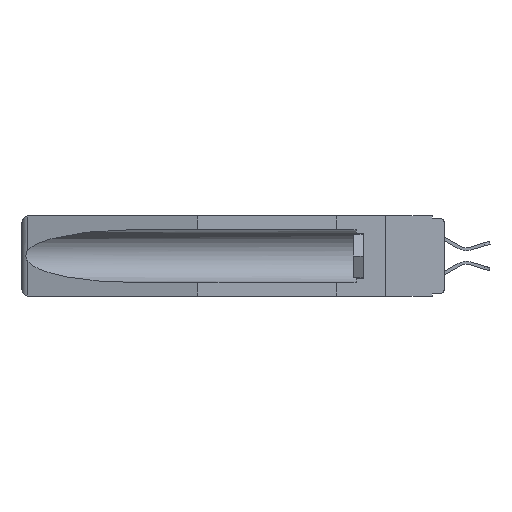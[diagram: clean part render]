
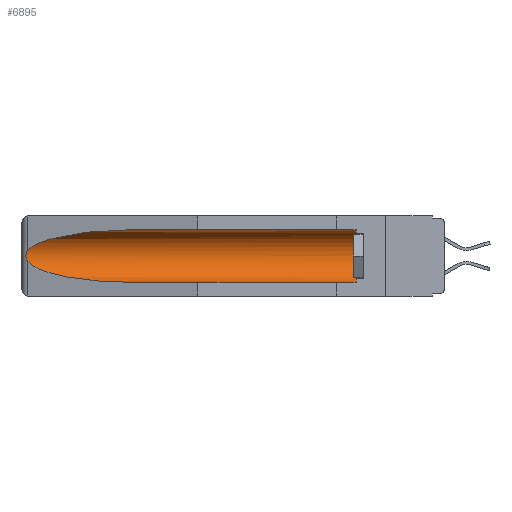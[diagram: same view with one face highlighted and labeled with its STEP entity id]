
A CAD part, left-side view. The second image highlights one B-rep face of the part: STEP entity #6895.
In plain terms, the highlighted cylindrical face has radius 2.857 mm (diameter 5.715 mm), a partial arc.
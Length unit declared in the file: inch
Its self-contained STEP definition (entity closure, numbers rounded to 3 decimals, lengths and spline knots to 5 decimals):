
#378 = CYLINDRICAL_SURFACE ( 'NONE', #2777, 0.1125 ) ;
#470 = CARTESIAN_POINT ( 'NONE',  ( 0.25451, 1.48313, -0.24835 ) ) ;
#1082 = CARTESIAN_POINT ( 'NONE',  ( 0.155, 0.126, -0.059 ) ) ;
#2229 = CARTESIAN_POINT ( 'NONE',  ( 0.26655, 1.53094, -0.18657 ) ) ;
#2641 = DIRECTION ( 'NONE',  ( 0., -1., 0. ) ) ;
#2777 = AXIS2_PLACEMENT_3D ( 'NONE', #6259, #7432, #11549 ) ;
#2891 = ORIENTED_EDGE ( 'NONE', *, *, #7883, .T. ) ;
#3202 = CARTESIAN_POINT ( 'NONE',  ( 0.25451, 1.48313, -0.09465 ) ) ;
#3220 = VERTEX_POINT ( 'NONE', #15635 ) ;
#3237 = ORIENTED_EDGE ( 'NONE', *, *, #11779, .T. ) ;
#3327 = EDGE_CURVE ( 'NONE', #3220, #6119, #5556, .T. ) ;
#3585 = CARTESIAN_POINT ( 'NONE',  ( 0.2675, 1.53308, -0.17534 ) ) ;
#3802 = VECTOR ( 'NONE', #13469, 39.37008 ) ;
#4016 = CARTESIAN_POINT ( 'NONE',  ( 0.155, 0.126, -0.1715 ) ) ;
#4204 = ORIENTED_EDGE ( 'NONE', *, *, #3327, .T. ) ;
#5072 = CARTESIAN_POINT ( 'NONE',  ( 0.26537, 1.52718, -0.19328 ) ) ;
#5439 = CARTESIAN_POINT ( 'NONE',  ( 0.155, 0.126, -0.284 ) ) ;
#5556 = B_SPLINE_CURVE_WITH_KNOTS ( 'NONE', 3,
 ( #6140, #10045, #17248, #13213, #15986, #3585, #10272, #2229, #15869, #5072 ),
 .UNSPECIFIED., .F., .F.,
 ( 4, 2, 2, 2, 4 ),
 ( 0., 0.00029, 0.00058, 0.00087, 0.00117 ),
 .UNSPECIFIED. ) ;
#5599 = ORIENTED_EDGE ( 'NONE', *, *, #7158, .T. ) ;
#5603 = EDGE_LOOP ( 'NONE', ( #3237, #4204, #2891, #5764, #15323, #5599 ) ) ;
#5764 = ORIENTED_EDGE ( 'NONE', *, *, #12818, .F. ) ;
#6076 = CARTESIAN_POINT ( 'NONE',  ( 0.26537, 1.52718, -0.19328 ) ) ;
#6119 = VERTEX_POINT ( 'NONE', #6076 ) ;
#6140 = CARTESIAN_POINT ( 'NONE',  ( 0.26537, 1.52718, -0.14972 ) ) ;
#6259 = CARTESIAN_POINT ( 'NONE',  ( 0.155, -0.30754, -0.1715 ) ) ;
#6714 = VERTEX_POINT ( 'NONE', #5439 ) ;
#6895 = ADVANCED_FACE ( 'NONE', ( #10347 ), #378, .F. ) ;
#7093 = AXIS2_PLACEMENT_3D ( 'NONE', #4016, #2641, #17561 ) ;
#7158 = EDGE_CURVE ( 'NONE', #10837, #15326, #8010, .T. ) ;
#7394 = LINE ( 'NONE', #9323, #3802 ) ;
#7432 = DIRECTION ( 'NONE',  ( 0., 1., 0. ) ) ;
#7724 = CARTESIAN_POINT ( 'NONE',  ( 0.155, 1.07973, -0.059 ) ) ;
#7883 = EDGE_CURVE ( 'NONE', #6119, #14030, #15288, .T. ) ;
#7953 = CARTESIAN_POINT ( 'NONE',  ( 0.155, -0.30754, -0.059 ) ) ;
#8010 = LINE ( 'NONE', #7953, #17233 ) ;
#8496 = CIRCLE ( 'NONE', #7093, 0.1125 ) ;
#9323 = CARTESIAN_POINT ( 'NONE',  ( 0.155, -0.30754, -0.284 ) ) ;
#10045 = CARTESIAN_POINT ( 'NONE',  ( 0.26597, 1.52961, -0.15275 ) ) ;
#10272 = CARTESIAN_POINT ( 'NONE',  ( 0.2673, 1.53269, -0.17917 ) ) ;
#10347 = FACE_OUTER_BOUND ( 'NONE', #5603, .T. ) ;
#10837 = VERTEX_POINT ( 'NONE', #1082 ) ;
#11337 = CARTESIAN_POINT ( 'NONE',  ( 0.155, 1.07973, -0.284 ) ) ;
#11549 = DIRECTION ( 'NONE',  ( 0., 0., 1. ) ) ;
#11779 = EDGE_CURVE ( 'NONE', #15326, #3220, #12072, .T. ) ;
#12072 =( BOUNDED_CURVE ( )  B_SPLINE_CURVE ( 3, ( #12899, #14044, #3202, #12724 ),
 .UNSPECIFIED., .F., .F. ) 
 B_SPLINE_CURVE_WITH_KNOTS ( ( 4, 4 ),
 ( 4.71239, 6.08839 ),
 .UNSPECIFIED. ) 
 CURVE ( )  GEOMETRIC_REPRESENTATION_ITEM ( )  RATIONAL_B_SPLINE_CURVE ( ( 1., 0.848, 0.848, 1. ) ) 
 REPRESENTATION_ITEM ( '' )  );
#12724 = CARTESIAN_POINT ( 'NONE',  ( 0.26537, 1.52718, -0.14972 ) ) ;
#12818 = EDGE_CURVE ( 'NONE', #6714, #14030, #7394, .T. ) ;
#12899 = CARTESIAN_POINT ( 'NONE',  ( 0.155, 1.07973, -0.059 ) ) ;
#12902 = CARTESIAN_POINT ( 'NONE',  ( 0.26537, 1.52718, -0.19328 ) ) ;
#13087 = CARTESIAN_POINT ( 'NONE',  ( 0.155, 1.07973, -0.284 ) ) ;
#13213 = CARTESIAN_POINT ( 'NONE',  ( 0.2673, 1.5327, -0.16383 ) ) ;
#13469 = DIRECTION ( 'NONE',  ( 0., 1., 0. ) ) ;
#14030 = VERTEX_POINT ( 'NONE', #13087 ) ;
#14044 = CARTESIAN_POINT ( 'NONE',  ( 0.21114, 1.30732, -0.059 ) ) ;
#14230 = CARTESIAN_POINT ( 'NONE',  ( 0.21114, 1.30732, -0.284 ) ) ;
#15288 =( BOUNDED_CURVE ( )  B_SPLINE_CURVE ( 3, ( #12902, #470, #14230, #11337 ),
 .UNSPECIFIED., .F., .F. ) 
 B_SPLINE_CURVE_WITH_KNOTS ( ( 4, 4 ),
 ( 0.1948, 1.5708 ),
 .UNSPECIFIED. ) 
 CURVE ( )  GEOMETRIC_REPRESENTATION_ITEM ( )  RATIONAL_B_SPLINE_CURVE ( ( 1., 0.848, 0.848, 1. ) ) 
 REPRESENTATION_ITEM ( '' )  );
#15323 = ORIENTED_EDGE ( 'NONE', *, *, #17278, .T. ) ;
#15326 = VERTEX_POINT ( 'NONE', #7724 ) ;
#15635 = CARTESIAN_POINT ( 'NONE',  ( 0.26537, 1.52718, -0.14972 ) ) ;
#15869 = CARTESIAN_POINT ( 'NONE',  ( 0.26597, 1.5296, -0.19026 ) ) ;
#15986 = CARTESIAN_POINT ( 'NONE',  ( 0.2675, 1.53308, -0.16763 ) ) ;
#16402 = DIRECTION ( 'NONE',  ( 0., 1., 0. ) ) ;
#17233 = VECTOR ( 'NONE', #16402, 39.37008 ) ;
#17248 = CARTESIAN_POINT ( 'NONE',  ( 0.26654, 1.53092, -0.15636 ) ) ;
#17278 = EDGE_CURVE ( 'NONE', #6714, #10837, #8496, .T. ) ;
#17561 = DIRECTION ( 'NONE',  ( 0., 0., 1. ) ) ;
